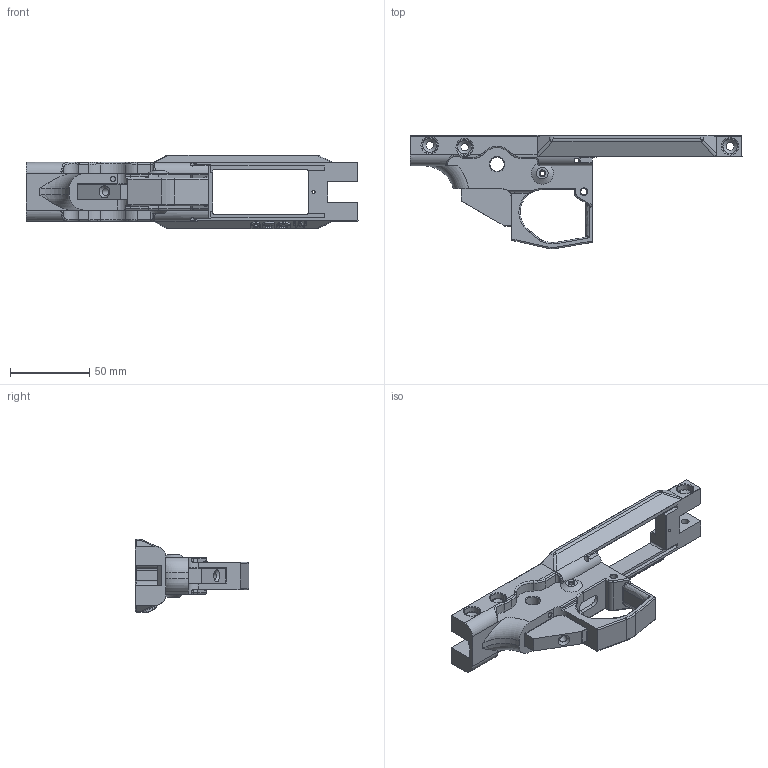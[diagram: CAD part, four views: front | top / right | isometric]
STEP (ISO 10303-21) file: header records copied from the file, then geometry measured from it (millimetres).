
FILE_DESCRIPTION(/* description */ (''),/* implementation_level */ '2;1');
FILE_NAME(/* name */ 'MOD9 LOWER 05 09 2020.stp',/* time_stamp */ '2020-09-05T20:23:01+03:00',/* author */ (''),/* organization */ (''),/* preprocessor_version */ 'ST-DEVELOPER v15.2',/* originating_system */ 'Autodesk Translator Framework v2.0.0.5431',/* authorisation */ '');
FILE_SCHEMA (('AUTOMOTIVE_DESIGN { 1 0 10303 214 3 1 1 }'));
Length unit declared in the file: centimetre
Products named in the file (1): goat mod9
Bounding box: 209 x 71.26 x 46.33 mm (x, y, z)
Volume: 101423.7 mm3; surface area: 40582.8 mm2
Topology: 1 solids, 2 shells, 546 faces, 1474 edges, 925 vertices
Faces by surface type: plane 176, bspline 150, cylinder 143, torus 39, cone 34, sphere 4
Full cylindrical faces by diameter (mm): 2 x1, 2.969 x4, 3.175 x1, 4 x1, 4.605 x1, 4.675 x2, 4.9 x2, 5.1 x2, 9.025 x2, 10 x6
Entity records: 23822 total; most frequent: CARTESIAN_POINT 11286, ORIENTED_EDGE 2818, DIRECTION 2192, EDGE_CURVE 1408, VERTEX_POINT 913, AXIS2_PLACEMENT_3D 757, LINE 678, VECTOR 678
